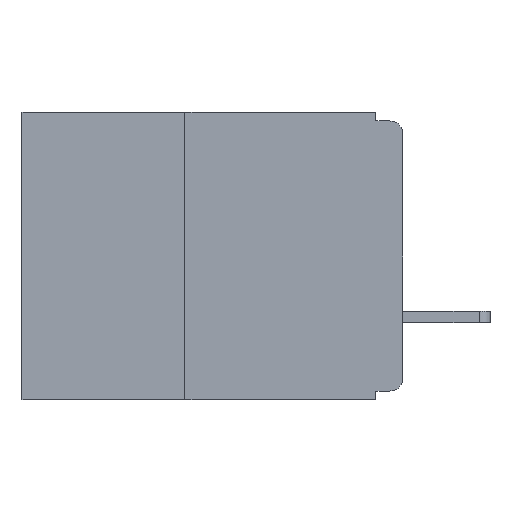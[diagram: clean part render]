
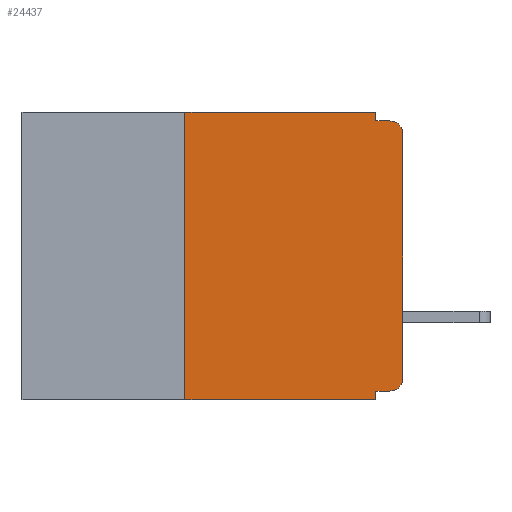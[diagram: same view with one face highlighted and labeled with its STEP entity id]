
A CAD part, left-side view. The second image highlights one B-rep face of the part: STEP entity #24437.
In plain terms, the highlighted planar face has unit normal (-1, 0, 0).
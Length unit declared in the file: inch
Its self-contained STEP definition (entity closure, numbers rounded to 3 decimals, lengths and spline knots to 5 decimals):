
#63 = EDGE_CURVE ( 'NONE', #12172, #32557, #20659, .T. ) ;
#450 = VERTEX_POINT ( 'NONE', #32452 ) ;
#678 = DIRECTION ( 'NONE',  ( 0., 0., -1. ) ) ;
#698 = CARTESIAN_POINT ( 'NONE',  ( 0., 0.031, 0. ) ) ;
#800 = EDGE_CURVE ( 'NONE', #29887, #450, #32810, .T. ) ;
#884 = EDGE_CURVE ( 'NONE', #26312, #14574, #17664, .T. ) ;
#1552 = ORIENTED_EDGE ( 'NONE', *, *, #27527, .F. ) ;
#1610 = ORIENTED_EDGE ( 'NONE', *, *, #884, .T. ) ;
#2132 = CARTESIAN_POINT ( 'NONE',  ( 0., 0.437, 0. ) ) ;
#2207 = CARTESIAN_POINT ( 'NONE',  ( 0., 0.25, -0.33 ) ) ;
#2254 = CARTESIAN_POINT ( 'NONE',  ( 0., 0.031, -0.33 ) ) ;
#2256 = CIRCLE ( 'NONE', #14849, 0.015 ) ;
#2830 = ORIENTED_EDGE ( 'NONE', *, *, #63, .F. ) ;
#3792 = EDGE_CURVE ( 'NONE', #12172, #26312, #2256, .T. ) ;
#3982 = VECTOR ( 'NONE', #24285, 39.37008 ) ;
#4518 = ORIENTED_EDGE ( 'NONE', *, *, #800, .T. ) ;
#6432 = CARTESIAN_POINT ( 'NONE',  ( 0., 0.015, -0.01 ) ) ;
#6906 = ORIENTED_EDGE ( 'NONE', *, *, #3792, .T. ) ;
#7033 = ORIENTED_EDGE ( 'NONE', *, *, #20373, .F. ) ;
#7148 = VECTOR ( 'NONE', #10300, 39.37008 ) ;
#8171 = ORIENTED_EDGE ( 'NONE', *, *, #11679, .T. ) ;
#8520 = CARTESIAN_POINT ( 'NONE',  ( 0., 0.25, 0. ) ) ;
#8656 = VECTOR ( 'NONE', #20137, 39.37008 ) ;
#9006 = PLANE ( 'NONE',  #25757 ) ;
#10300 = DIRECTION ( 'NONE',  ( 0., 0., 1. ) ) ;
#10710 = EDGE_CURVE ( 'NONE', #16367, #23992, #14713, .T. ) ;
#10836 = LINE ( 'NONE', #698, #3982 ) ;
#11304 = CARTESIAN_POINT ( 'NONE',  ( 0., 0.031, -0.32 ) ) ;
#11328 = CARTESIAN_POINT ( 'NONE',  ( 0., 0.015, -0.025 ) ) ;
#11679 = EDGE_CURVE ( 'NONE', #14574, #23992, #25495, .T. ) ;
#11707 = LINE ( 'NONE', #2254, #17687 ) ;
#12172 = VERTEX_POINT ( 'NONE', #18731 ) ;
#12183 = CARTESIAN_POINT ( 'NONE',  ( 0., 0., -0.305 ) ) ;
#13898 = DIRECTION ( 'NONE',  ( 0., 0., -1. ) ) ;
#13934 = VECTOR ( 'NONE', #28097, 39.37008 ) ;
#14047 = CARTESIAN_POINT ( 'NONE',  ( 0., 0.031, -0.01 ) ) ;
#14200 = DIRECTION ( 'NONE',  ( 0., 0., -1. ) ) ;
#14235 = CARTESIAN_POINT ( 'NONE',  ( 0., 0., -0.025 ) ) ;
#14239 = CARTESIAN_POINT ( 'NONE',  ( 0., 0.031, 0. ) ) ;
#14526 = EDGE_CURVE ( 'NONE', #17094, #16367, #10836, .T. ) ;
#14574 = VERTEX_POINT ( 'NONE', #14235 ) ;
#14713 = LINE ( 'NONE', #17623, #8656 ) ;
#14849 = AXIS2_PLACEMENT_3D ( 'NONE', #29061, #24865, #678 ) ;
#14961 = CARTESIAN_POINT ( 'NONE',  ( 0., 0.437, -0.33 ) ) ;
#15132 = ORIENTED_EDGE ( 'NONE', *, *, #32260, .F. ) ;
#16220 = CARTESIAN_POINT ( 'NONE',  ( 0., 0., 0. ) ) ;
#16367 = VERTEX_POINT ( 'NONE', #14047 ) ;
#17094 = VERTEX_POINT ( 'NONE', #14239 ) ;
#17622 = DIRECTION ( 'NONE',  ( 0., 0., -1. ) ) ;
#17623 = CARTESIAN_POINT ( 'NONE',  ( 0., 0., -0.01 ) ) ;
#17664 = LINE ( 'NONE', #16220, #23669 ) ;
#17687 = VECTOR ( 'NONE', #17622, 39.37008 ) ;
#17829 = VECTOR ( 'NONE', #20014, 39.37008 ) ;
#18731 = CARTESIAN_POINT ( 'NONE',  ( 0., 0.015, -0.32 ) ) ;
#20014 = DIRECTION ( 'NONE',  ( 0., -1., 0. ) ) ;
#20137 = DIRECTION ( 'NONE',  ( 0., -1., 0. ) ) ;
#20373 = EDGE_CURVE ( 'NONE', #32557, #450, #11707, .T. ) ;
#20659 = LINE ( 'NONE', #28137, #13934 ) ;
#20824 = ORIENTED_EDGE ( 'NONE', *, *, #10710, .F. ) ;
#21537 = LINE ( 'NONE', #30735, #7148 ) ;
#21979 = EDGE_LOOP ( 'NONE', ( #1610, #8171, #20824, #24389, #1552, #15132, #4518, #7033, #2830, #6906 ) ) ;
#22032 = DIRECTION ( 'NONE',  ( 0., 0., 1. ) ) ;
#23042 = AXIS2_PLACEMENT_3D ( 'NONE', #11328, #29176, #13898 ) ;
#23669 = VECTOR ( 'NONE', #22032, 39.37008 ) ;
#23992 = VERTEX_POINT ( 'NONE', #6432 ) ;
#24285 = DIRECTION ( 'NONE',  ( 0., 0., -1. ) ) ;
#24389 = ORIENTED_EDGE ( 'NONE', *, *, #14526, .F. ) ;
#24437 = ADVANCED_FACE ( 'NONE', ( #29044 ), #9006, .F. ) ;
#24643 = LINE ( 'NONE', #2132, #17829 ) ;
#24865 = DIRECTION ( 'NONE',  ( -1., 0., 0. ) ) ;
#25495 = CIRCLE ( 'NONE', #23042, 0.015 ) ;
#25757 = AXIS2_PLACEMENT_3D ( 'NONE', #26926, #29471, #14200 ) ;
#26104 = VECTOR ( 'NONE', #26799, 39.37008 ) ;
#26312 = VERTEX_POINT ( 'NONE', #12183 ) ;
#26799 = DIRECTION ( 'NONE',  ( 0., -1., 0. ) ) ;
#26926 = CARTESIAN_POINT ( 'NONE',  ( 0., 0.437, 0. ) ) ;
#27527 = EDGE_CURVE ( 'NONE', #29527, #17094, #24643, .T. ) ;
#28097 = DIRECTION ( 'NONE',  ( 0., 1., 0. ) ) ;
#28137 = CARTESIAN_POINT ( 'NONE',  ( 0., 0., -0.32 ) ) ;
#29044 = FACE_OUTER_BOUND ( 'NONE', #21979, .T. ) ;
#29061 = CARTESIAN_POINT ( 'NONE',  ( 0., 0.015, -0.305 ) ) ;
#29176 = DIRECTION ( 'NONE',  ( -1., 0., 0. ) ) ;
#29471 = DIRECTION ( 'NONE',  ( 1., 0., 0. ) ) ;
#29527 = VERTEX_POINT ( 'NONE', #8520 ) ;
#29887 = VERTEX_POINT ( 'NONE', #2207 ) ;
#30735 = CARTESIAN_POINT ( 'NONE',  ( 0., 0.25, -0.33 ) ) ;
#32260 = EDGE_CURVE ( 'NONE', #29887, #29527, #21537, .T. ) ;
#32452 = CARTESIAN_POINT ( 'NONE',  ( 0., 0.031, -0.33 ) ) ;
#32557 = VERTEX_POINT ( 'NONE', #11304 ) ;
#32810 = LINE ( 'NONE', #14961, #26104 ) ;
